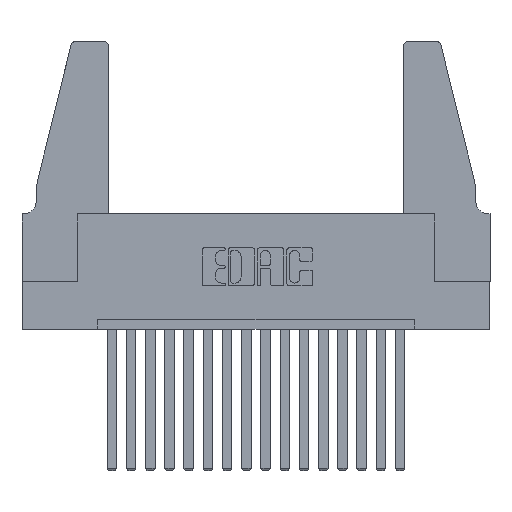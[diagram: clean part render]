
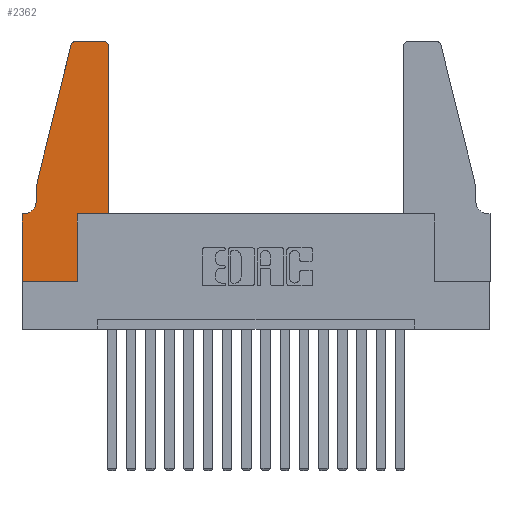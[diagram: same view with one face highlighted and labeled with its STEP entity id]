
A CAD part, top view. The second image highlights one B-rep face of the part: STEP entity #2362.
In plain terms, the highlighted planar face has unit normal (0, 0, 1).
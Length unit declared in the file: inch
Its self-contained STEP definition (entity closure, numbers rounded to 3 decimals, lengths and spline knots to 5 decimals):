
#214 = DIRECTION ( 'NONE',  ( 0., 0., 1. ) ) ;
#325 = CARTESIAN_POINT ( 'NONE',  ( 0.2865, 0.35, 0.37 ) ) ;
#704 = CARTESIAN_POINT ( 'NONE',  ( 0.4505, 0.35, 0.37 ) ) ;
#826 = EDGE_CURVE ( 'NONE', #13664, #2091, #12623, .T. ) ;
#899 = CARTESIAN_POINT ( 'NONE',  ( 0.4505, 1.22, 0.37 ) ) ;
#915 = EDGE_CURVE ( 'NONE', #16501, #14598, #11775, .T. ) ;
#1040 = CARTESIAN_POINT ( 'NONE',  ( 0.2605, 1.25, 0.37 ) ) ;
#1170 = ORIENTED_EDGE ( 'NONE', *, *, #16758, .T. ) ;
#1367 = AXIS2_PLACEMENT_3D ( 'NONE', #6787, #12197, #16166 ) ;
#1411 = VERTEX_POINT ( 'NONE', #3957 ) ;
#1436 = ORIENTED_EDGE ( 'NONE', *, *, #1818, .T. ) ;
#1636 = EDGE_CURVE ( 'NONE', #14598, #7485, #3762, .T. ) ;
#1673 = LINE ( 'NONE', #325, #11590 ) ;
#1808 = CARTESIAN_POINT ( 'NONE',  ( 0.25487, 1.22718, 0.37 ) ) ;
#1818 = EDGE_CURVE ( 'NONE', #7726, #7478, #16197, .T. ) ;
#2075 = DIRECTION ( 'NONE',  ( -1., 0., 0. ) ) ;
#2091 = VERTEX_POINT ( 'NONE', #13693 ) ;
#2228 = LINE ( 'NONE', #1040, #8792 ) ;
#2362 = ADVANCED_FACE ( 'NONE', ( #7126 ), #2956, .T. ) ;
#2479 = CIRCLE ( 'NONE', #17049, 0.03 ) ;
#2665 = EDGE_LOOP ( 'NONE', ( #12716, #12020, #17269, #17018, #11880, #12982, #6220, #9797, #5253, #1436, #8782, #1170 ) ) ;
#2956 = PLANE ( 'NONE',  #15429 ) ;
#2960 = CARTESIAN_POINT ( 'NONE',  ( 0.0755, 0.42, 0.37 ) ) ;
#3762 = LINE ( 'NONE', #15524, #8181 ) ;
#3798 = DIRECTION ( 'NONE',  ( 0., 0., 1. ) ) ;
#3957 = CARTESIAN_POINT ( 'NONE',  ( 0.0755, 0.5, 0.37 ) ) ;
#3971 = DIRECTION ( 'NONE',  ( 0., -1., 0. ) ) ;
#4147 = CIRCLE ( 'NONE', #12631, 0.03 ) ;
#4975 = CARTESIAN_POINT ( 'NONE',  ( 0.4505, 0.35, 0.37 ) ) ;
#5072 = DIRECTION ( 'NONE',  ( 0., 0., 1. ) ) ;
#5189 = CARTESIAN_POINT ( 'NONE',  ( 0.0755, 0.5, 0.37 ) ) ;
#5246 = DIRECTION ( 'NONE',  ( 1., 0., 0. ) ) ;
#5253 = ORIENTED_EDGE ( 'NONE', *, *, #12745, .T. ) ;
#5300 = CARTESIAN_POINT ( 'NONE',  ( 0.2865, 0.35, 0.37 ) ) ;
#5662 = VECTOR ( 'NONE', #15855, 39.37008 ) ;
#6127 = CARTESIAN_POINT ( 'NONE',  ( 0.4505, 0.35, 0.37 ) ) ;
#6220 = ORIENTED_EDGE ( 'NONE', *, *, #16788, .T. ) ;
#6306 = CARTESIAN_POINT ( 'NONE',  ( 0.284, 1.25, 0.37 ) ) ;
#6504 = DIRECTION ( 'NONE',  ( -1., 0., 0. ) ) ;
#6550 = CARTESIAN_POINT ( 'NONE',  ( 0., 0., 0.37 ) ) ;
#6787 = CARTESIAN_POINT ( 'NONE',  ( 0.0055, 0.42, 0.37 ) ) ;
#6901 = LINE ( 'NONE', #704, #10056 ) ;
#7125 = CARTESIAN_POINT ( 'NONE',  ( 0.0755, 0.5, 0.37 ) ) ;
#7126 = FACE_OUTER_BOUND ( 'NONE', #2665, .T. ) ;
#7242 = VERTEX_POINT ( 'NONE', #14942 ) ;
#7478 = VERTEX_POINT ( 'NONE', #4975 ) ;
#7485 = VERTEX_POINT ( 'NONE', #14419 ) ;
#7726 = VERTEX_POINT ( 'NONE', #5300 ) ;
#7818 = CARTESIAN_POINT ( 'NONE',  ( 0., 0., 0.37 ) ) ;
#8110 = CARTESIAN_POINT ( 'NONE',  ( 0., 0.35, 0.37 ) ) ;
#8181 = VECTOR ( 'NONE', #2075, 39.37008 ) ;
#8388 = EDGE_CURVE ( 'NONE', #7478, #11000, #6901, .T. ) ;
#8576 = CARTESIAN_POINT ( 'NONE',  ( 0.0055, 0.35, 0.37 ) ) ;
#8782 = ORIENTED_EDGE ( 'NONE', *, *, #8388, .T. ) ;
#8792 = VECTOR ( 'NONE', #6504, 39.37008 ) ;
#9012 = VECTOR ( 'NONE', #12895, 39.37008 ) ;
#9270 = VECTOR ( 'NONE', #13267, 39.37008 ) ;
#9797 = ORIENTED_EDGE ( 'NONE', *, *, #826, .T. ) ;
#10056 = VECTOR ( 'NONE', #11451, 39.37008 ) ;
#10977 = VERTEX_POINT ( 'NONE', #6306 ) ;
#11000 = VERTEX_POINT ( 'NONE', #899 ) ;
#11263 = DIRECTION ( 'NONE',  ( 0., -1., 0. ) ) ;
#11292 = LINE ( 'NONE', #7818, #14489 ) ;
#11340 = LINE ( 'NONE', #5189, #5662 ) ;
#11451 = DIRECTION ( 'NONE',  ( 0., 1., 0. ) ) ;
#11590 = VECTOR ( 'NONE', #15044, 39.37008 ) ;
#11775 = CIRCLE ( 'NONE', #1367, 0.07 ) ;
#11849 = CARTESIAN_POINT ( 'NONE',  ( 0.4205, 1.22, 0.37 ) ) ;
#11880 = ORIENTED_EDGE ( 'NONE', *, *, #915, .T. ) ;
#12020 = ORIENTED_EDGE ( 'NONE', *, *, #15616, .T. ) ;
#12197 = DIRECTION ( 'NONE',  ( 0., 0., -1. ) ) ;
#12623 = LINE ( 'NONE', #6550, #9270 ) ;
#12631 = AXIS2_PLACEMENT_3D ( 'NONE', #11849, #3798, #13221 ) ;
#12716 = ORIENTED_EDGE ( 'NONE', *, *, #16699, .T. ) ;
#12745 = EDGE_CURVE ( 'NONE', #2091, #7726, #1673, .T. ) ;
#12800 = LINE ( 'NONE', #7125, #16405 ) ;
#12895 = DIRECTION ( 'NONE',  ( 1., 0., 0. ) ) ;
#12982 = ORIENTED_EDGE ( 'NONE', *, *, #1636, .T. ) ;
#13221 = DIRECTION ( 'NONE',  ( 1., 0., 0. ) ) ;
#13267 = DIRECTION ( 'NONE',  ( 1., 0., 0. ) ) ;
#13664 = VERTEX_POINT ( 'NONE', #13728 ) ;
#13693 = CARTESIAN_POINT ( 'NONE',  ( 0.2865, 0., 0.37 ) ) ;
#13728 = CARTESIAN_POINT ( 'NONE',  ( 0., 0., 0.37 ) ) ;
#14419 = CARTESIAN_POINT ( 'NONE',  ( 0., 0.35, 0.37 ) ) ;
#14489 = VECTOR ( 'NONE', #3971, 39.37008 ) ;
#14593 = EDGE_CURVE ( 'NONE', #1411, #16501, #12800, .T. ) ;
#14598 = VERTEX_POINT ( 'NONE', #8576 ) ;
#14942 = CARTESIAN_POINT ( 'NONE',  ( 0.4205, 1.25, 0.37 ) ) ;
#14996 = DIRECTION ( 'NONE',  ( 1., 0., 0. ) ) ;
#15044 = DIRECTION ( 'NONE',  ( 0., 1., 0. ) ) ;
#15429 = AXIS2_PLACEMENT_3D ( 'NONE', #8110, #214, #14996 ) ;
#15524 = CARTESIAN_POINT ( 'NONE',  ( 0.0755, 0.35, 0.37 ) ) ;
#15599 = EDGE_CURVE ( 'NONE', #17488, #1411, #11340, .T. ) ;
#15616 = EDGE_CURVE ( 'NONE', #10977, #17488, #2479, .T. ) ;
#15855 = DIRECTION ( 'NONE',  ( -0.239, -0.971, 0. ) ) ;
#15912 = CARTESIAN_POINT ( 'NONE',  ( 0.284, 1.22, 0.37 ) ) ;
#16166 = DIRECTION ( 'NONE',  ( -1., 0., 0. ) ) ;
#16197 = LINE ( 'NONE', #6127, #9012 ) ;
#16405 = VECTOR ( 'NONE', #11263, 39.37008 ) ;
#16501 = VERTEX_POINT ( 'NONE', #2960 ) ;
#16699 = EDGE_CURVE ( 'NONE', #7242, #10977, #2228, .T. ) ;
#16758 = EDGE_CURVE ( 'NONE', #11000, #7242, #4147, .T. ) ;
#16788 = EDGE_CURVE ( 'NONE', #7485, #13664, #11292, .T. ) ;
#17018 = ORIENTED_EDGE ( 'NONE', *, *, #14593, .T. ) ;
#17049 = AXIS2_PLACEMENT_3D ( 'NONE', #15912, #5072, #5246 ) ;
#17269 = ORIENTED_EDGE ( 'NONE', *, *, #15599, .T. ) ;
#17488 = VERTEX_POINT ( 'NONE', #1808 ) ;
